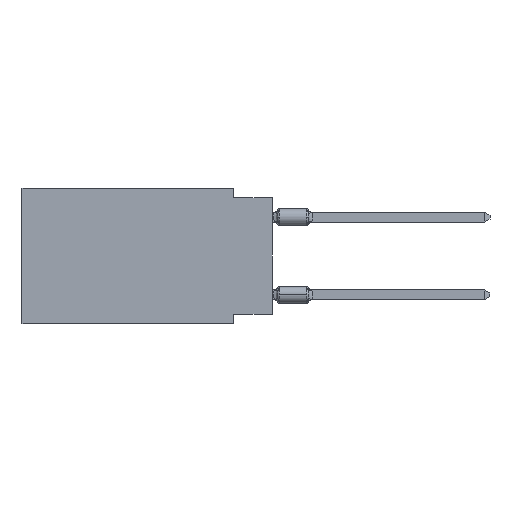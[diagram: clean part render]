
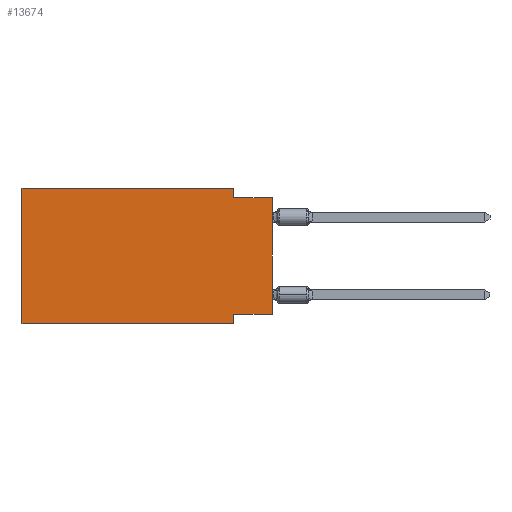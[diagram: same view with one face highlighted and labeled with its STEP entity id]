
A CAD part, left-side view. The second image highlights one B-rep face of the part: STEP entity #13674.
In plain terms, the highlighted planar face has unit normal (-1, 0, 0).
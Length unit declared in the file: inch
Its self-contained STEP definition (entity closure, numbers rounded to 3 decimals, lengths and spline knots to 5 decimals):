
#672 = VECTOR ( 'NONE', #8517, 39.37008 ) ;
#901 = EDGE_CURVE ( 'NONE', #9940, #9405, #911, .T. ) ;
#911 = LINE ( 'NONE', #12759, #9868 ) ;
#1160 = CARTESIAN_POINT ( 'NONE',  ( 0., 0.1, 0. ) ) ;
#1343 = ORIENTED_EDGE ( 'NONE', *, *, #13082, .F. ) ;
#1562 = CARTESIAN_POINT ( 'NONE',  ( 0., 0.645, 0. ) ) ;
#1593 = EDGE_CURVE ( 'NONE', #4562, #8418, #9328, .T. ) ;
#1617 = CARTESIAN_POINT ( 'NONE',  ( 0., 0., -0.025 ) ) ;
#1685 = LINE ( 'NONE', #2539, #672 ) ;
#1820 = ORIENTED_EDGE ( 'NONE', *, *, #901, .F. ) ;
#2034 = DIRECTION ( 'NONE',  ( 0., 1., 0. ) ) ;
#2140 = EDGE_CURVE ( 'NONE', #4562, #8427, #1685, .T. ) ;
#2310 = VECTOR ( 'NONE', #7103, 39.37008 ) ;
#2501 = ORIENTED_EDGE ( 'NONE', *, *, #8025, .F. ) ;
#2539 = CARTESIAN_POINT ( 'NONE',  ( 0., 0., 0. ) ) ;
#2595 = CARTESIAN_POINT ( 'NONE',  ( 0., 0.1, -0.35 ) ) ;
#3483 = AXIS2_PLACEMENT_3D ( 'NONE', #12127, #6166, #3945 ) ;
#3945 = DIRECTION ( 'NONE',  ( 0., 0., -1. ) ) ;
#4052 = CARTESIAN_POINT ( 'NONE',  ( 0., 0.1, -0.35 ) ) ;
#4533 = LINE ( 'NONE', #9371, #9611 ) ;
#4562 = VERTEX_POINT ( 'NONE', #7520 ) ;
#5211 = VECTOR ( 'NONE', #2034, 39.37008 ) ;
#5283 = ORIENTED_EDGE ( 'NONE', *, *, #6237, .F. ) ;
#5366 = VERTEX_POINT ( 'NONE', #1160 ) ;
#5748 = DIRECTION ( 'NONE',  ( 0., 0., -1. ) ) ;
#5880 = ORIENTED_EDGE ( 'NONE', *, *, #11786, .T. ) ;
#6166 = DIRECTION ( 'NONE',  ( 1., 0., 0. ) ) ;
#6237 = EDGE_CURVE ( 'NONE', #10117, #8427, #12014, .T. ) ;
#6242 = FACE_OUTER_BOUND ( 'NONE', #9131, .T. ) ;
#6776 = CARTESIAN_POINT ( 'NONE',  ( 0., 0., -0.025 ) ) ;
#7010 = CARTESIAN_POINT ( 'NONE',  ( 0., 0.1, -0.325 ) ) ;
#7103 = DIRECTION ( 'NONE',  ( 0., -1., 0. ) ) ;
#7520 = CARTESIAN_POINT ( 'NONE',  ( 0., 0., -0.325 ) ) ;
#7626 = DIRECTION ( 'NONE',  ( 0., 0., -1. ) ) ;
#7868 = LINE ( 'NONE', #4052, #13550 ) ;
#8025 = EDGE_CURVE ( 'NONE', #9405, #5366, #11689, .T. ) ;
#8094 = VERTEX_POINT ( 'NONE', #2595 ) ;
#8418 = VERTEX_POINT ( 'NONE', #7010 ) ;
#8427 = VERTEX_POINT ( 'NONE', #6776 ) ;
#8517 = DIRECTION ( 'NONE',  ( 0., 0., 1. ) ) ;
#9131 = EDGE_LOOP ( 'NONE', ( #10984, #5283, #1343, #2501, #1820, #5880, #9556, #11423 ) ) ;
#9199 = DIRECTION ( 'NONE',  ( 0., 0., 1. ) ) ;
#9328 = LINE ( 'NONE', #14045, #5211 ) ;
#9371 = CARTESIAN_POINT ( 'NONE',  ( 0., 0.1, 0. ) ) ;
#9405 = VERTEX_POINT ( 'NONE', #1562 ) ;
#9556 = ORIENTED_EDGE ( 'NONE', *, *, #14795, .F. ) ;
#9611 = VECTOR ( 'NONE', #5748, 39.37008 ) ;
#9659 = VECTOR ( 'NONE', #9683, 39.37008 ) ;
#9683 = DIRECTION ( 'NONE',  ( 0., -1., 0. ) ) ;
#9714 = PLANE ( 'NONE',  #3483 ) ;
#9868 = VECTOR ( 'NONE', #9199, 39.37008 ) ;
#9940 = VERTEX_POINT ( 'NONE', #12753 ) ;
#10117 = VERTEX_POINT ( 'NONE', #12131 ) ;
#10350 = CARTESIAN_POINT ( 'NONE',  ( 0., 0.645, 0. ) ) ;
#10388 = VECTOR ( 'NONE', #12191, 39.37008 ) ;
#10984 = ORIENTED_EDGE ( 'NONE', *, *, #2140, .T. ) ;
#11423 = ORIENTED_EDGE ( 'NONE', *, *, #1593, .F. ) ;
#11689 = LINE ( 'NONE', #10350, #2310 ) ;
#11786 = EDGE_CURVE ( 'NONE', #9940, #8094, #12263, .T. ) ;
#12014 = LINE ( 'NONE', #1617, #9659 ) ;
#12127 = CARTESIAN_POINT ( 'NONE',  ( 0., 0.645, 0. ) ) ;
#12131 = CARTESIAN_POINT ( 'NONE',  ( 0., 0.1, -0.025 ) ) ;
#12191 = DIRECTION ( 'NONE',  ( 0., -1., 0. ) ) ;
#12263 = LINE ( 'NONE', #14875, #10388 ) ;
#12753 = CARTESIAN_POINT ( 'NONE',  ( 0., 0.645, -0.35 ) ) ;
#12759 = CARTESIAN_POINT ( 'NONE',  ( 0., 0.645, 0. ) ) ;
#13082 = EDGE_CURVE ( 'NONE', #5366, #10117, #4533, .T. ) ;
#13550 = VECTOR ( 'NONE', #7626, 39.37008 ) ;
#13674 = ADVANCED_FACE ( 'NONE', ( #6242 ), #9714, .F. ) ;
#14045 = CARTESIAN_POINT ( 'NONE',  ( 0., 0., -0.325 ) ) ;
#14795 = EDGE_CURVE ( 'NONE', #8418, #8094, #7868, .T. ) ;
#14875 = CARTESIAN_POINT ( 'NONE',  ( 0., 0.645, -0.35 ) ) ;
